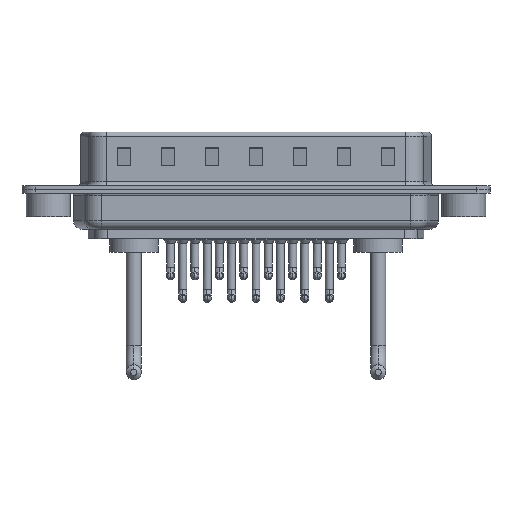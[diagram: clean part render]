
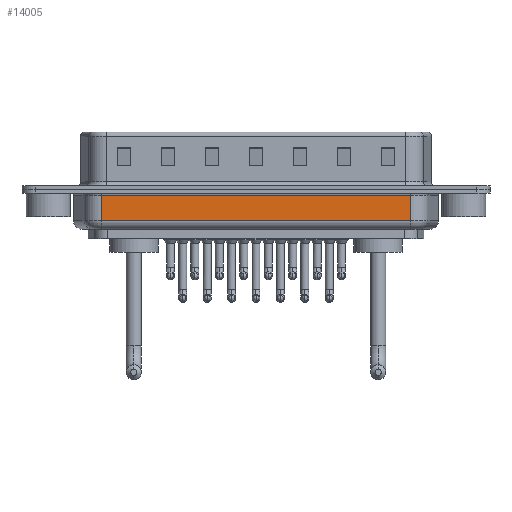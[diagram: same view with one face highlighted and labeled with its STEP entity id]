
A CAD part, front view. The second image highlights one B-rep face of the part: STEP entity #14005.
In plain terms, the highlighted planar face has unit normal (0, -1, 0).
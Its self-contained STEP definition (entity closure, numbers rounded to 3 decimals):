
#872 = ORIENTED_EDGE ( 'NONE', *, *, #9875, .T. ) ;
#1534 = CARTESIAN_POINT ( 'NONE',  ( 6.006, -5.35, -3.5 ) ) ;
#1695 = AXIS2_PLACEMENT_3D ( 'NONE', #17503, #22899, #7355 ) ;
#1952 = DIRECTION ( 'NONE',  ( 0., 0., 1. ) ) ;
#2349 = VECTOR ( 'NONE', #3475, 1000. ) ;
#2394 = ORIENTED_EDGE ( 'NONE', *, *, #15451, .T. ) ;
#2889 = DIRECTION ( 'NONE',  ( -1., 0., 0. ) ) ;
#3326 = EDGE_LOOP ( 'NONE', ( #24480, #2394, #872, #12502 ) ) ;
#3475 = DIRECTION ( 'NONE',  ( 0., 0., 1. ) ) ;
#5141 = CARTESIAN_POINT ( 'NONE',  ( 6.006, -5.35, -0.65 ) ) ;
#7355 = DIRECTION ( 'NONE',  ( 0., 0., 1. ) ) ;
#7602 = PLANE ( 'NONE',  #1695 ) ;
#7982 = VERTEX_POINT ( 'NONE', #21514 ) ;
#8143 = EDGE_CURVE ( 'NONE', #21484, #20052, #9225, .T. ) ;
#9225 = LINE ( 'NONE', #20994, #17939 ) ;
#9875 = EDGE_CURVE ( 'NONE', #7982, #12842, #18789, .T. ) ;
#12411 = EDGE_CURVE ( 'NONE', #12842, #20052, #22311, .T. ) ;
#12502 = ORIENTED_EDGE ( 'NONE', *, *, #12411, .T. ) ;
#12842 = VERTEX_POINT ( 'NONE', #23676 ) ;
#14005 = ADVANCED_FACE ( 'NONE', ( #15132 ), #7602, .F. ) ;
#15132 = FACE_OUTER_BOUND ( 'NONE', #3326, .T. ) ;
#15451 = EDGE_CURVE ( 'NONE', #21484, #7982, #20612, .T. ) ;
#17503 = CARTESIAN_POINT ( 'NONE',  ( 6.006, -5.35, -4.5 ) ) ;
#17939 = VECTOR ( 'NONE', #1952, 1000. ) ;
#18789 = LINE ( 'NONE', #19040, #2349 ) ;
#19040 = CARTESIAN_POINT ( 'NONE',  ( 41.044, -5.35, -4.5 ) ) ;
#20052 = VERTEX_POINT ( 'NONE', #24488 ) ;
#20612 = LINE ( 'NONE', #22119, #24133 ) ;
#20865 = VECTOR ( 'NONE', #2889, 1000. ) ;
#20994 = CARTESIAN_POINT ( 'NONE',  ( 6.006, -5.35, -4.5 ) ) ;
#21484 = VERTEX_POINT ( 'NONE', #1534 ) ;
#21514 = CARTESIAN_POINT ( 'NONE',  ( 41.044, -5.35, -3.5 ) ) ;
#22119 = CARTESIAN_POINT ( 'NONE',  ( 6.006, -5.35, -3.5 ) ) ;
#22311 = LINE ( 'NONE', #5141, #20865 ) ;
#22899 = DIRECTION ( 'NONE',  ( 0., 1., 0. ) ) ;
#23676 = CARTESIAN_POINT ( 'NONE',  ( 41.044, -5.35, -0.65 ) ) ;
#24129 = DIRECTION ( 'NONE',  ( 1., 0., 0. ) ) ;
#24133 = VECTOR ( 'NONE', #24129, 1000. ) ;
#24480 = ORIENTED_EDGE ( 'NONE', *, *, #8143, .F. ) ;
#24488 = CARTESIAN_POINT ( 'NONE',  ( 6.006, -5.35, -0.65 ) ) ;
